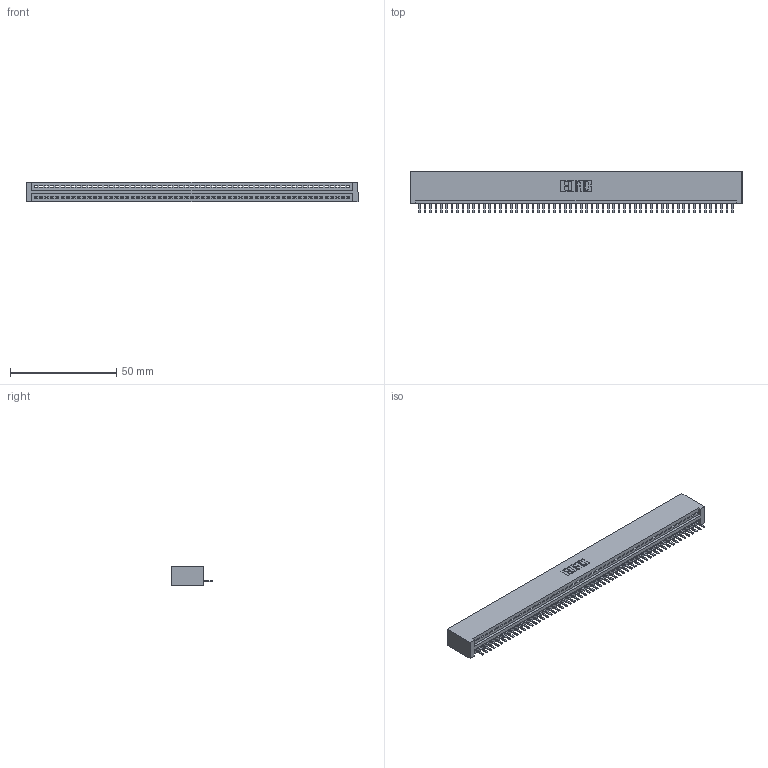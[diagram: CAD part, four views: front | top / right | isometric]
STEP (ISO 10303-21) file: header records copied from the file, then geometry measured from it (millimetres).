
FILE_DESCRIPTION (( 'STEP AP203' ), '1' );
FILE_NAME ('345-059-520-101.STEP', '2018-09-26T19:11:29', ( '' ), ( '' ), 'SwSTEP 2.0', 'SolidWorks 2016', '' );
FILE_SCHEMA (( 'CONFIG_CONTROL_DESIGN' ));
Length unit declared in the file: inch
Products named in the file (3): 345-292-001_345-293-120; 345-059-520-101; 345 Part_No Mounting Lugs
Assembly tree (60 placements, depth 2):
  345-059-520-101
    345 Part_No Mounting Lugs
    345-292-001_345-293-120  x59
Bounding box: 156.46 x 19.68 x 9.4 mm (x, y, z)
Volume: 15415 mm3; surface area: 20351.1 mm2
Topology: 60 solids, 60 shells, 3776 faces, 11173 edges, 7290 vertices
Faces by surface type: plane 2554, cylinder 1222
Entity records: 41953 total; most frequent: CARTESIAN_POINT 7285, ORIENTED_EDGE 7266, DIRECTION 6319, EDGE_CURVE 3633, LINE 3269, VECTOR 3269, VERTEX_POINT 2418, AXIS2_PLACEMENT_3D 1525
